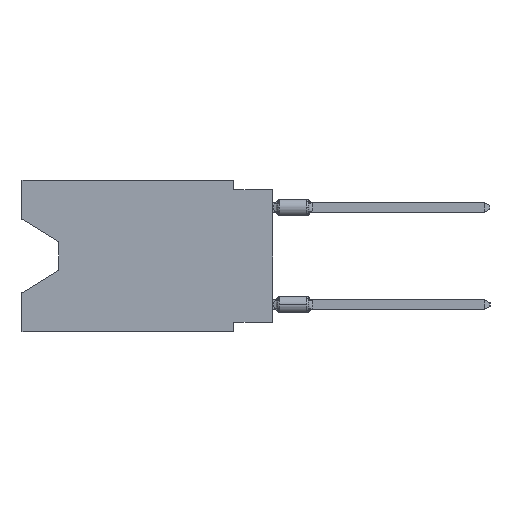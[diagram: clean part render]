
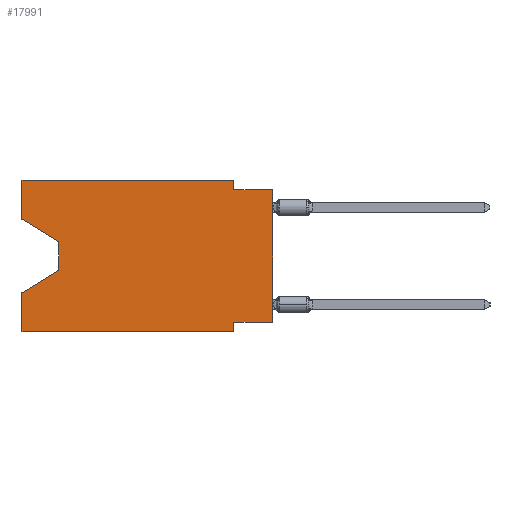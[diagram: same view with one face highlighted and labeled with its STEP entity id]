
A CAD part, left-side view. The second image highlights one B-rep face of the part: STEP entity #17991.
In plain terms, the highlighted planar face has unit normal (-1, 0, 0).
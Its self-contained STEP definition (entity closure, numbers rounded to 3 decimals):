
#531 = LINE ( 'NONE', #4566, #5160 ) ;
#3114 = CARTESIAN_POINT ( 'NONE',  ( 0., 16.383, 0. ) ) ;
#4566 = CARTESIAN_POINT ( 'NONE',  ( 0., 13.97, -5.893 ) ) ;
#5160 = VECTOR ( 'NONE', #25008, 1000. ) ;
#5215 = VECTOR ( 'NONE', #34023, 1000. ) ;
#6768 = ORIENTED_EDGE ( 'NONE', *, *, #29504, .T. ) ;
#7358 = VECTOR ( 'NONE', #38553, 1000. ) ;
#7506 = VECTOR ( 'NONE', #43502, 1000. ) ;
#7700 = ORIENTED_EDGE ( 'NONE', *, *, #61363, .F. ) ;
#9520 = ORIENTED_EDGE ( 'NONE', *, *, #51889, .T. ) ;
#9948 = CARTESIAN_POINT ( 'NONE',  ( 0., 16.383, 0. ) ) ;
#11447 = VECTOR ( 'NONE', #59741, 1000. ) ;
#11889 = CARTESIAN_POINT ( 'NONE',  ( 0., 13.97, -4.013 ) ) ;
#14143 = EDGE_CURVE ( 'NONE', #19921, #27889, #27753, .T. ) ;
#14959 = CARTESIAN_POINT ( 'NONE',  ( 0., 2.54, -9.906 ) ) ;
#15201 = AXIS2_PLACEMENT_3D ( 'NONE', #18404, #54941, #54263 ) ;
#15643 = ORIENTED_EDGE ( 'NONE', *, *, #40564, .F. ) ;
#16364 = CARTESIAN_POINT ( 'NONE',  ( 0., 16.383, 0. ) ) ;
#16527 = VERTEX_POINT ( 'NONE', #46259 ) ;
#17991 = ADVANCED_FACE ( 'NONE', ( #48573 ), #28127, .F. ) ;
#18404 = CARTESIAN_POINT ( 'NONE',  ( 0., 16.383, 0. ) ) ;
#18603 = VECTOR ( 'NONE', #43480, 1000. ) ;
#19113 = CARTESIAN_POINT ( 'NONE',  ( 0., 2.54, 0. ) ) ;
#19921 = VERTEX_POINT ( 'NONE', #19113 ) ;
#20663 = CARTESIAN_POINT ( 'NONE',  ( 0., 16.383, -2.546 ) ) ;
#20878 = VERTEX_POINT ( 'NONE', #51082 ) ;
#21228 = CARTESIAN_POINT ( 'NONE',  ( 0., 2.54, -0.635 ) ) ;
#22744 = EDGE_LOOP ( 'NONE', ( #31337, #9520, #34372, #15643, #43972, #7700, #40909, #6768, #61857, #41449, #39712, #37608 ) ) ;
#23288 = DIRECTION ( 'NONE',  ( 0., 0., -1. ) ) ;
#24703 = DIRECTION ( 'NONE',  ( 0., 0., 1. ) ) ;
#25008 = DIRECTION ( 'NONE',  ( 0., 0.855, -0.519 ) ) ;
#25417 = VERTEX_POINT ( 'NONE', #20663 ) ;
#25717 = VECTOR ( 'NONE', #24703, 1000. ) ;
#25742 = LINE ( 'NONE', #61273, #40952 ) ;
#25950 = VERTEX_POINT ( 'NONE', #40873 ) ;
#27753 = LINE ( 'NONE', #37473, #7506 ) ;
#27889 = VERTEX_POINT ( 'NONE', #21228 ) ;
#28053 = EDGE_CURVE ( 'NONE', #49699, #19921, #64101, .T. ) ;
#28127 = PLANE ( 'NONE',  #15201 ) ;
#28785 = VERTEX_POINT ( 'NONE', #31774 ) ;
#29504 = EDGE_CURVE ( 'NONE', #34245, #25950, #51634, .T. ) ;
#29805 = EDGE_CURVE ( 'NONE', #32452, #16527, #44581, .T. ) ;
#30625 = CARTESIAN_POINT ( 'NONE',  ( 0., 16.383, -7.36 ) ) ;
#31019 = EDGE_CURVE ( 'NONE', #25417, #49699, #37032, .T. ) ;
#31337 = ORIENTED_EDGE ( 'NONE', *, *, #36353, .T. ) ;
#31774 = CARTESIAN_POINT ( 'NONE',  ( 0., 13.97, -4.013 ) ) ;
#32452 = VERTEX_POINT ( 'NONE', #47036 ) ;
#33327 = LINE ( 'NONE', #11889, #50259 ) ;
#34023 = DIRECTION ( 'NONE',  ( 0., 0., 1. ) ) ;
#34245 = VERTEX_POINT ( 'NONE', #62716 ) ;
#34372 = ORIENTED_EDGE ( 'NONE', *, *, #65695, .T. ) ;
#34868 = DIRECTION ( 'NONE',  ( 0., 1., 0. ) ) ;
#36353 = EDGE_CURVE ( 'NONE', #25417, #28785, #58580, .T. ) ;
#36975 = VECTOR ( 'NONE', #41405, 1000. ) ;
#37032 = LINE ( 'NONE', #38385, #65283 ) ;
#37473 = CARTESIAN_POINT ( 'NONE',  ( 0., 2.54, 0. ) ) ;
#37608 = ORIENTED_EDGE ( 'NONE', *, *, #31019, .F. ) ;
#38385 = CARTESIAN_POINT ( 'NONE',  ( 0., 16.383, 0. ) ) ;
#38553 = DIRECTION ( 'NONE',  ( 0., -1., 0. ) ) ;
#39712 = ORIENTED_EDGE ( 'NONE', *, *, #28053, .F. ) ;
#40408 = VECTOR ( 'NONE', #34868, 1000. ) ;
#40564 = EDGE_CURVE ( 'NONE', #32452, #44499, #55879, .T. ) ;
#40873 = CARTESIAN_POINT ( 'NONE',  ( 0., 0., -0.635 ) ) ;
#40909 = ORIENTED_EDGE ( 'NONE', *, *, #63411, .F. ) ;
#40952 = VECTOR ( 'NONE', #51859, 1000. ) ;
#41405 = DIRECTION ( 'NONE',  ( 0., 0., -1. ) ) ;
#41449 = ORIENTED_EDGE ( 'NONE', *, *, #14143, .F. ) ;
#42484 = CARTESIAN_POINT ( 'NONE',  ( 0., 16.383, -2.546 ) ) ;
#43480 = DIRECTION ( 'NONE',  ( 0., -0.855, -0.519 ) ) ;
#43502 = DIRECTION ( 'NONE',  ( 0., 0., -1. ) ) ;
#43954 = CARTESIAN_POINT ( 'NONE',  ( 0., 0., -9.271 ) ) ;
#43972 = ORIENTED_EDGE ( 'NONE', *, *, #29805, .T. ) ;
#44080 = CARTESIAN_POINT ( 'NONE',  ( 0., 0., 0. ) ) ;
#44499 = VERTEX_POINT ( 'NONE', #30625 ) ;
#44581 = LINE ( 'NONE', #64033, #7358 ) ;
#46259 = CARTESIAN_POINT ( 'NONE',  ( 0., 2.54, -9.906 ) ) ;
#46534 = CARTESIAN_POINT ( 'NONE',  ( 0., 13.97, -5.893 ) ) ;
#47036 = CARTESIAN_POINT ( 'NONE',  ( 0., 16.383, -9.906 ) ) ;
#48573 = FACE_OUTER_BOUND ( 'NONE', #22744, .T. ) ;
#49699 = VERTEX_POINT ( 'NONE', #16364 ) ;
#50259 = VECTOR ( 'NONE', #23288, 1000. ) ;
#51082 = CARTESIAN_POINT ( 'NONE',  ( 0., 2.54, -9.271 ) ) ;
#51634 = LINE ( 'NONE', #44080, #5215 ) ;
#51859 = DIRECTION ( 'NONE',  ( 0., -1., 0. ) ) ;
#51889 = EDGE_CURVE ( 'NONE', #28785, #52590, #33327, .T. ) ;
#52590 = VERTEX_POINT ( 'NONE', #46534 ) ;
#54263 = DIRECTION ( 'NONE',  ( 0., 0., -1. ) ) ;
#54941 = DIRECTION ( 'NONE',  ( 1., 0., 0. ) ) ;
#55879 = LINE ( 'NONE', #9948, #25717 ) ;
#56225 = EDGE_CURVE ( 'NONE', #27889, #25950, #25742, .T. ) ;
#56524 = LINE ( 'NONE', #14959, #36975 ) ;
#58580 = LINE ( 'NONE', #42484, #18603 ) ;
#58830 = DIRECTION ( 'NONE',  ( 0., 0., 1. ) ) ;
#59036 = LINE ( 'NONE', #43954, #40408 ) ;
#59741 = DIRECTION ( 'NONE',  ( 0., -1., 0. ) ) ;
#61273 = CARTESIAN_POINT ( 'NONE',  ( 0., 0., -0.635 ) ) ;
#61363 = EDGE_CURVE ( 'NONE', #20878, #16527, #56524, .T. ) ;
#61857 = ORIENTED_EDGE ( 'NONE', *, *, #56225, .F. ) ;
#62716 = CARTESIAN_POINT ( 'NONE',  ( 0., 0., -9.271 ) ) ;
#63411 = EDGE_CURVE ( 'NONE', #34245, #20878, #59036, .T. ) ;
#64033 = CARTESIAN_POINT ( 'NONE',  ( 0., 16.383, -9.906 ) ) ;
#64101 = LINE ( 'NONE', #3114, #11447 ) ;
#65283 = VECTOR ( 'NONE', #58830, 1000. ) ;
#65695 = EDGE_CURVE ( 'NONE', #52590, #44499, #531, .T. ) ;
